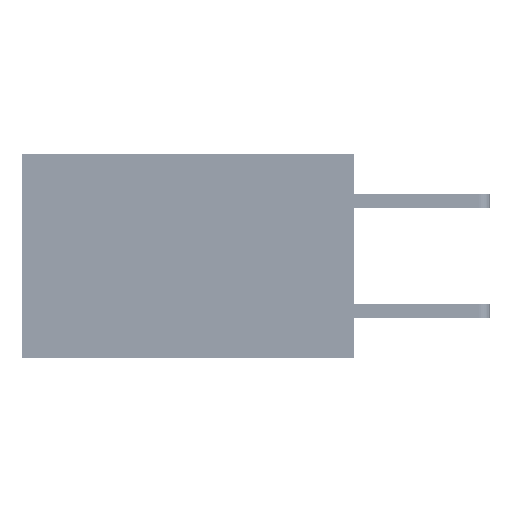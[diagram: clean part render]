
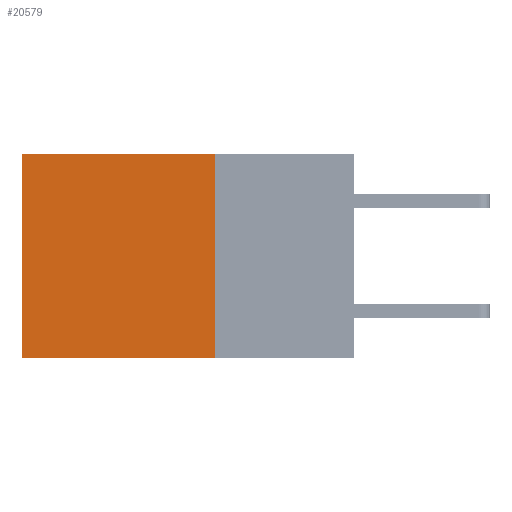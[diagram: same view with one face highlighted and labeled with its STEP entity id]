
A CAD part, left-side view. The second image highlights one B-rep face of the part: STEP entity #20579.
In plain terms, the highlighted planar face has unit normal (-1, 0, 0).
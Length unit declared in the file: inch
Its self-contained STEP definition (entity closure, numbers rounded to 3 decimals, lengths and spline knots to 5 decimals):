
#636 = VERTEX_POINT ( 'NONE', #16809 ) ;
#2063 = CARTESIAN_POINT ( 'NONE',  ( 0.2875, 0.6, -0.37 ) ) ;
#5063 = EDGE_LOOP ( 'NONE', ( #33856, #12627, #13770, #5691 ) ) ;
#5691 = ORIENTED_EDGE ( 'NONE', *, *, #20300, .T. ) ;
#7480 = CARTESIAN_POINT ( 'NONE',  ( 0.2875, 0.25, -0.37 ) ) ;
#7618 = DIRECTION ( 'NONE',  ( 0., 1., 0. ) ) ;
#8780 = LINE ( 'NONE', #9227, #39096 ) ;
#9227 = CARTESIAN_POINT ( 'NONE',  ( 0.2875, 0.25, 0. ) ) ;
#9505 = LINE ( 'NONE', #34197, #17689 ) ;
#12084 = CARTESIAN_POINT ( 'NONE',  ( 0.2875, 0.25, 0. ) ) ;
#12627 = ORIENTED_EDGE ( 'NONE', *, *, #30881, .F. ) ;
#12783 = FACE_OUTER_BOUND ( 'NONE', #5063, .T. ) ;
#13551 = CARTESIAN_POINT ( 'NONE',  ( 0.2875, 0.25, 0. ) ) ;
#13770 = ORIENTED_EDGE ( 'NONE', *, *, #30819, .F. ) ;
#14255 = AXIS2_PLACEMENT_3D ( 'NONE', #12084, #27681, #15391 ) ;
#15391 = DIRECTION ( 'NONE',  ( 0., 0., -1. ) ) ;
#16143 = LINE ( 'NONE', #13551, #34152 ) ;
#16809 = CARTESIAN_POINT ( 'NONE',  ( 0.2875, 0.25, -0.37 ) ) ;
#17689 = VECTOR ( 'NONE', #22474, 39.37008 ) ;
#19668 = DIRECTION ( 'NONE',  ( 0., 1., 0. ) ) ;
#20300 = EDGE_CURVE ( 'NONE', #32093, #32578, #16143, .T. ) ;
#20579 = ADVANCED_FACE ( 'NONE', ( #12783 ), #30062, .F. ) ;
#21045 = VERTEX_POINT ( 'NONE', #2063 ) ;
#22474 = DIRECTION ( 'NONE',  ( 0., 0., -1. ) ) ;
#25400 = LINE ( 'NONE', #7480, #35789 ) ;
#25933 = EDGE_CURVE ( 'NONE', #32578, #21045, #9505, .T. ) ;
#27524 = CARTESIAN_POINT ( 'NONE',  ( 0.2875, 0.6, 0. ) ) ;
#27681 = DIRECTION ( 'NONE',  ( 1., 0., 0. ) ) ;
#30062 = PLANE ( 'NONE',  #14255 ) ;
#30819 = EDGE_CURVE ( 'NONE', #32093, #636, #8780, .T. ) ;
#30881 = EDGE_CURVE ( 'NONE', #636, #21045, #25400, .T. ) ;
#32093 = VERTEX_POINT ( 'NONE', #37695 ) ;
#32578 = VERTEX_POINT ( 'NONE', #27524 ) ;
#33856 = ORIENTED_EDGE ( 'NONE', *, *, #25933, .T. ) ;
#34152 = VECTOR ( 'NONE', #19668, 39.37008 ) ;
#34197 = CARTESIAN_POINT ( 'NONE',  ( 0.2875, 0.6, 0. ) ) ;
#35789 = VECTOR ( 'NONE', #7618, 39.37008 ) ;
#36403 = DIRECTION ( 'NONE',  ( 0., 0., -1. ) ) ;
#37695 = CARTESIAN_POINT ( 'NONE',  ( 0.2875, 0.25, 0. ) ) ;
#39096 = VECTOR ( 'NONE', #36403, 39.37008 ) ;
